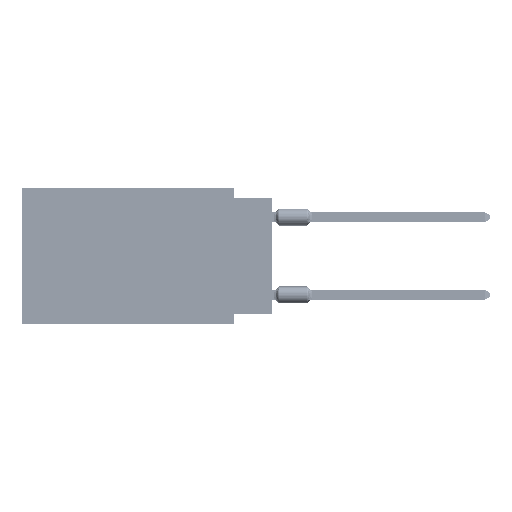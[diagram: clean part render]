
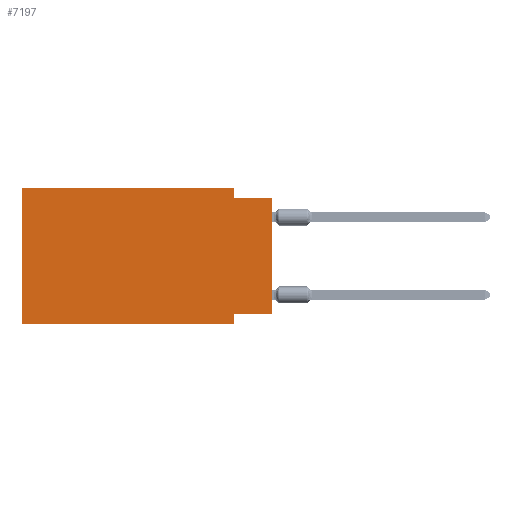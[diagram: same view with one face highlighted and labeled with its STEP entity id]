
A CAD part, left-side view. The second image highlights one B-rep face of the part: STEP entity #7197.
In plain terms, the highlighted planar face has unit normal (-1, 0, 0).
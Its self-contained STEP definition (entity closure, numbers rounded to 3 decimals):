
#5639 = VERTEX_POINT ( 'NONE', #25932 ) ;
#5989 = CARTESIAN_POINT ( 'NONE',  ( 0., 2.54, 0. ) ) ;
#6076 = VECTOR ( 'NONE', #42505, 1000. ) ;
#6248 = FACE_OUTER_BOUND ( 'NONE', #16562, .T. ) ;
#6760 = EDGE_CURVE ( 'NONE', #18416, #5639, #37454, .T. ) ;
#6933 = LINE ( 'NONE', #63369, #6076 ) ;
#7197 = ADVANCED_FACE ( 'NONE', ( #6248 ), #42507, .F. ) ;
#8012 = DIRECTION ( 'NONE',  ( 0., 0., 1. ) ) ;
#11385 = DIRECTION ( 'NONE',  ( 1., 0., 0. ) ) ;
#11460 = DIRECTION ( 'NONE',  ( 0., 0., -1. ) ) ;
#11958 = CARTESIAN_POINT ( 'NONE',  ( 0., 0., 0. ) ) ;
#13900 = CARTESIAN_POINT ( 'NONE',  ( 0., 2.54, 0. ) ) ;
#13919 = CARTESIAN_POINT ( 'NONE',  ( 0., 16.383, 0. ) ) ;
#13945 = EDGE_CURVE ( 'NONE', #5639, #29827, #6933, .T. ) ;
#14254 = ORIENTED_EDGE ( 'NONE', *, *, #20755, .F. ) ;
#14299 = CARTESIAN_POINT ( 'NONE',  ( 0., 2.54, -8.89 ) ) ;
#14725 = CARTESIAN_POINT ( 'NONE',  ( 0., 16.383, 0. ) ) ;
#16562 = EDGE_LOOP ( 'NONE', ( #54794, #44886, #34355, #14254, #58892, #54715, #58868, #29466 ) ) ;
#18416 = VERTEX_POINT ( 'NONE', #13900 ) ;
#19133 = DIRECTION ( 'NONE',  ( 0., 1., 0. ) ) ;
#20755 = EDGE_CURVE ( 'NONE', #48512, #18416, #33411, .T. ) ;
#22925 = LINE ( 'NONE', #60520, #47535 ) ;
#24091 = LINE ( 'NONE', #35013, #32634 ) ;
#24388 = CARTESIAN_POINT ( 'NONE',  ( 0., 2.54, -8.89 ) ) ;
#25071 = VECTOR ( 'NONE', #11460, 1000. ) ;
#25530 = VERTEX_POINT ( 'NONE', #63736 ) ;
#25784 = EDGE_CURVE ( 'NONE', #53154, #35334, #42707, .T. ) ;
#25932 = CARTESIAN_POINT ( 'NONE',  ( 0., 2.54, -0.635 ) ) ;
#27329 = DIRECTION ( 'NONE',  ( 0., -1., 0. ) ) ;
#28881 = EDGE_CURVE ( 'NONE', #25530, #29827, #37940, .T. ) ;
#29085 = VECTOR ( 'NONE', #56833, 1000. ) ;
#29466 = ORIENTED_EDGE ( 'NONE', *, *, #65823, .F. ) ;
#29827 = VERTEX_POINT ( 'NONE', #57777 ) ;
#32634 = VECTOR ( 'NONE', #8012, 1000. ) ;
#33411 = LINE ( 'NONE', #13919, #66824 ) ;
#34355 = ORIENTED_EDGE ( 'NONE', *, *, #6760, .F. ) ;
#35013 = CARTESIAN_POINT ( 'NONE',  ( 0., 16.383, 0. ) ) ;
#35334 = VERTEX_POINT ( 'NONE', #14299 ) ;
#37454 = LINE ( 'NONE', #5989, #25071 ) ;
#37940 = LINE ( 'NONE', #11958, #67603 ) ;
#38703 = VERTEX_POINT ( 'NONE', #47716 ) ;
#42505 = DIRECTION ( 'NONE',  ( 0., -1., 0. ) ) ;
#42507 = PLANE ( 'NONE',  #46928 ) ;
#42707 = LINE ( 'NONE', #45897, #56220 ) ;
#44886 = ORIENTED_EDGE ( 'NONE', *, *, #13945, .F. ) ;
#45897 = CARTESIAN_POINT ( 'NONE',  ( 0., 16.383, -8.89 ) ) ;
#46928 = AXIS2_PLACEMENT_3D ( 'NONE', #58227, #11385, #52753 ) ;
#47535 = VECTOR ( 'NONE', #19133, 1000. ) ;
#47716 = CARTESIAN_POINT ( 'NONE',  ( 0., 2.54, -8.255 ) ) ;
#48512 = VERTEX_POINT ( 'NONE', #14725 ) ;
#51763 = EDGE_CURVE ( 'NONE', #38703, #35334, #55494, .T. ) ;
#52753 = DIRECTION ( 'NONE',  ( 0., 0., -1. ) ) ;
#53154 = VERTEX_POINT ( 'NONE', #54373 ) ;
#54264 = DIRECTION ( 'NONE',  ( 0., -1., 0. ) ) ;
#54334 = DIRECTION ( 'NONE',  ( 0., 0., 1. ) ) ;
#54373 = CARTESIAN_POINT ( 'NONE',  ( 0., 16.383, -8.89 ) ) ;
#54715 = ORIENTED_EDGE ( 'NONE', *, *, #25784, .T. ) ;
#54794 = ORIENTED_EDGE ( 'NONE', *, *, #28881, .T. ) ;
#55494 = LINE ( 'NONE', #24388, #29085 ) ;
#56220 = VECTOR ( 'NONE', #27329, 1000. ) ;
#56603 = EDGE_CURVE ( 'NONE', #53154, #48512, #24091, .T. ) ;
#56833 = DIRECTION ( 'NONE',  ( 0., 0., -1. ) ) ;
#57777 = CARTESIAN_POINT ( 'NONE',  ( 0., 0., -0.635 ) ) ;
#58227 = CARTESIAN_POINT ( 'NONE',  ( 0., 16.383, 0. ) ) ;
#58868 = ORIENTED_EDGE ( 'NONE', *, *, #51763, .F. ) ;
#58892 = ORIENTED_EDGE ( 'NONE', *, *, #56603, .F. ) ;
#60520 = CARTESIAN_POINT ( 'NONE',  ( 0., 0., -8.255 ) ) ;
#63369 = CARTESIAN_POINT ( 'NONE',  ( 0., 0., -0.635 ) ) ;
#63736 = CARTESIAN_POINT ( 'NONE',  ( 0., 0., -8.255 ) ) ;
#65823 = EDGE_CURVE ( 'NONE', #25530, #38703, #22925, .T. ) ;
#66824 = VECTOR ( 'NONE', #54264, 1000. ) ;
#67603 = VECTOR ( 'NONE', #54334, 1000. ) ;
